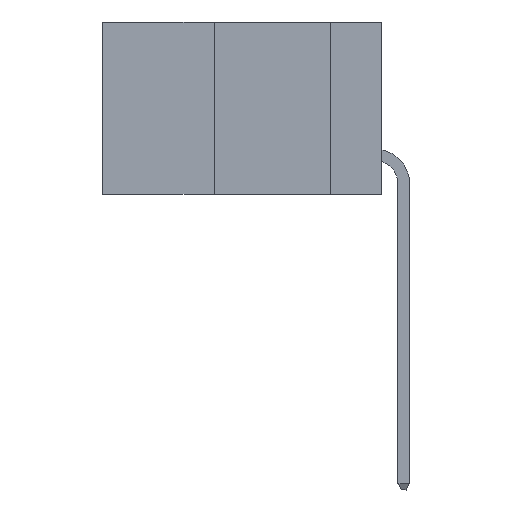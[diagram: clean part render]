
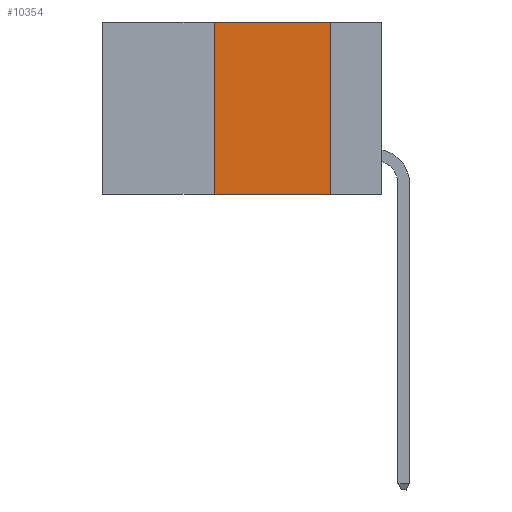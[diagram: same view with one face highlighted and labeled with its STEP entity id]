
A CAD part, left-side view. The second image highlights one B-rep face of the part: STEP entity #10354.
In plain terms, the highlighted planar face has unit normal (-1, 0, 0).
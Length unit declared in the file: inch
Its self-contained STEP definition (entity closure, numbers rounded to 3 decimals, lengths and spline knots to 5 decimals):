
#221 = CARTESIAN_POINT ( 'NONE',  ( 0., 0.36, -0.37 ) ) ;
#753 = CARTESIAN_POINT ( 'NONE',  ( 0., 0.6, 0. ) ) ;
#946 = AXIS2_PLACEMENT_3D ( 'NONE', #12370, #7664, #11295 ) ;
#1726 = VERTEX_POINT ( 'NONE', #6855 ) ;
#2711 = VECTOR ( 'NONE', #13913, 39.37008 ) ;
#2888 = VECTOR ( 'NONE', #6492, 39.37008 ) ;
#2955 = LINE ( 'NONE', #3092, #11367 ) ;
#3092 = CARTESIAN_POINT ( 'NONE',  ( 0., 0.6, -0.37 ) ) ;
#3235 = VERTEX_POINT ( 'NONE', #5548 ) ;
#3502 = CARTESIAN_POINT ( 'NONE',  ( 0., 0.11, 0. ) ) ;
#4434 = CARTESIAN_POINT ( 'NONE',  ( 0., 0.36, 0. ) ) ;
#4580 = LINE ( 'NONE', #753, #2711 ) ;
#4752 = ORIENTED_EDGE ( 'NONE', *, *, #13275, .T. ) ;
#4855 = ORIENTED_EDGE ( 'NONE', *, *, #6871, .F. ) ;
#5280 = ORIENTED_EDGE ( 'NONE', *, *, #8569, .F. ) ;
#5410 = PLANE ( 'NONE',  #946 ) ;
#5548 = CARTESIAN_POINT ( 'NONE',  ( 0., 0.36, 0. ) ) ;
#5582 = LINE ( 'NONE', #4434, #2888 ) ;
#5764 = EDGE_LOOP ( 'NONE', ( #14187, #4855, #5280, #4752 ) ) ;
#6492 = DIRECTION ( 'NONE',  ( 0., 0., 1. ) ) ;
#6559 = VECTOR ( 'NONE', #13432, 39.37008 ) ;
#6855 = CARTESIAN_POINT ( 'NONE',  ( 0., 0.11, -0.37 ) ) ;
#6871 = EDGE_CURVE ( 'NONE', #3235, #12971, #4580, .T. ) ;
#7504 = LINE ( 'NONE', #12130, #6559 ) ;
#7664 = DIRECTION ( 'NONE',  ( 1., 0., 0. ) ) ;
#8569 = EDGE_CURVE ( 'NONE', #12868, #3235, #5582, .T. ) ;
#9848 = DIRECTION ( 'NONE',  ( 0., -1., 0. ) ) ;
#10354 = ADVANCED_FACE ( 'NONE', ( #14631 ), #5410, .F. ) ;
#11295 = DIRECTION ( 'NONE',  ( 0., 0., -1. ) ) ;
#11367 = VECTOR ( 'NONE', #9848, 39.37008 ) ;
#12130 = CARTESIAN_POINT ( 'NONE',  ( 0., 0.11, 0. ) ) ;
#12370 = CARTESIAN_POINT ( 'NONE',  ( 0., 0.6, 0. ) ) ;
#12868 = VERTEX_POINT ( 'NONE', #221 ) ;
#12971 = VERTEX_POINT ( 'NONE', #3502 ) ;
#13275 = EDGE_CURVE ( 'NONE', #12868, #1726, #2955, .T. ) ;
#13432 = DIRECTION ( 'NONE',  ( 0., 0., -1. ) ) ;
#13913 = DIRECTION ( 'NONE',  ( 0., -1., 0. ) ) ;
#14187 = ORIENTED_EDGE ( 'NONE', *, *, #14611, .F. ) ;
#14611 = EDGE_CURVE ( 'NONE', #12971, #1726, #7504, .T. ) ;
#14631 = FACE_OUTER_BOUND ( 'NONE', #5764, .T. ) ;
